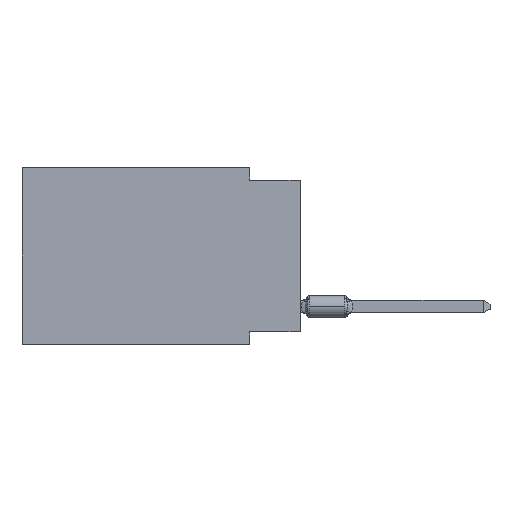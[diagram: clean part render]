
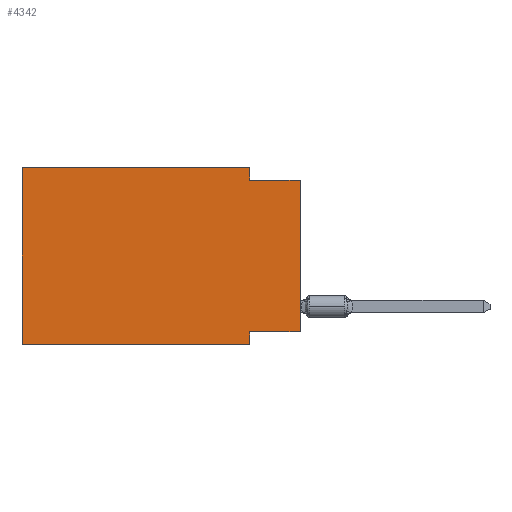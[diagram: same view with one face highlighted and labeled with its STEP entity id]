
A CAD part, left-side view. The second image highlights one B-rep face of the part: STEP entity #4342.
In plain terms, the highlighted planar face has unit normal (-1, 0, 0).
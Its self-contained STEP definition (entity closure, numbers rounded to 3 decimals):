
#394 = CARTESIAN_POINT ( 'NONE',  ( 0., 13.97, 0. ) ) ;
#446 = DIRECTION ( 'NONE',  ( 0., 1., 0. ) ) ;
#1307 = LINE ( 'NONE', #6825, #6203 ) ;
#1561 = DIRECTION ( 'NONE',  ( 0., 0., -1. ) ) ;
#2312 = CARTESIAN_POINT ( 'NONE',  ( 0., 0., -0.635 ) ) ;
#2677 = CARTESIAN_POINT ( 'NONE',  ( 0., 0., 0. ) ) ;
#3046 = EDGE_LOOP ( 'NONE', ( #17296, #5006, #12104, #15900, #17443, #9702, #17251, #3530 ) ) ;
#3286 = DIRECTION ( 'NONE',  ( 0., -1., 0. ) ) ;
#3456 = VECTOR ( 'NONE', #1561, 1000. ) ;
#3530 = ORIENTED_EDGE ( 'NONE', *, *, #16984, .F. ) ;
#3575 = CARTESIAN_POINT ( 'NONE',  ( 0., 2.54, -8.89 ) ) ;
#3631 = VERTEX_POINT ( 'NONE', #10836 ) ;
#3987 = VERTEX_POINT ( 'NONE', #11901 ) ;
#4277 = CARTESIAN_POINT ( 'NONE',  ( 0., 2.54, 0. ) ) ;
#4342 = ADVANCED_FACE ( 'NONE', ( #6666 ), #5301, .F. ) ;
#4349 = CARTESIAN_POINT ( 'NONE',  ( 0., 0., -8.255 ) ) ;
#4372 = VERTEX_POINT ( 'NONE', #14952 ) ;
#4436 = EDGE_CURVE ( 'NONE', #3631, #6353, #15126, .T. ) ;
#4737 = LINE ( 'NONE', #2312, #9221 ) ;
#4914 = VERTEX_POINT ( 'NONE', #13649 ) ;
#5006 = ORIENTED_EDGE ( 'NONE', *, *, #14986, .F. ) ;
#5114 = LINE ( 'NONE', #3575, #11708 ) ;
#5301 = PLANE ( 'NONE',  #11368 ) ;
#6203 = VECTOR ( 'NONE', #12318, 1000. ) ;
#6353 = VERTEX_POINT ( 'NONE', #12789 ) ;
#6480 = DIRECTION ( 'NONE',  ( 0., 0., -1. ) ) ;
#6558 = CARTESIAN_POINT ( 'NONE',  ( 0., 13.97, 0. ) ) ;
#6666 = FACE_OUTER_BOUND ( 'NONE', #3046, .T. ) ;
#6825 = CARTESIAN_POINT ( 'NONE',  ( 0., 13.97, -8.89 ) ) ;
#7093 = EDGE_CURVE ( 'NONE', #7919, #4914, #1307, .T. ) ;
#7183 = EDGE_CURVE ( 'NONE', #15101, #3987, #10141, .T. ) ;
#7353 = CARTESIAN_POINT ( 'NONE',  ( 0., 13.97, 0. ) ) ;
#7648 = LINE ( 'NONE', #4349, #14333 ) ;
#7919 = VERTEX_POINT ( 'NONE', #17100 ) ;
#7927 = VECTOR ( 'NONE', #8531, 1000. ) ;
#8531 = DIRECTION ( 'NONE',  ( 0., 0., 1. ) ) ;
#8983 = EDGE_CURVE ( 'NONE', #15997, #4914, #5114, .T. ) ;
#9221 = VECTOR ( 'NONE', #17374, 1000. ) ;
#9653 = CARTESIAN_POINT ( 'NONE',  ( 0., 2.54, -8.255 ) ) ;
#9702 = ORIENTED_EDGE ( 'NONE', *, *, #7093, .T. ) ;
#10141 = LINE ( 'NONE', #394, #17426 ) ;
#10621 = CARTESIAN_POINT ( 'NONE',  ( 0., 13.97, 0. ) ) ;
#10836 = CARTESIAN_POINT ( 'NONE',  ( 0., 0., -8.255 ) ) ;
#11368 = AXIS2_PLACEMENT_3D ( 'NONE', #10621, #17573, #6480 ) ;
#11708 = VECTOR ( 'NONE', #14495, 1000. ) ;
#11716 = EDGE_CURVE ( 'NONE', #7919, #15101, #17089, .T. ) ;
#11901 = CARTESIAN_POINT ( 'NONE',  ( 0., 2.54, 0. ) ) ;
#11951 = EDGE_CURVE ( 'NONE', #3987, #4372, #12483, .T. ) ;
#12104 = ORIENTED_EDGE ( 'NONE', *, *, #11951, .F. ) ;
#12318 = DIRECTION ( 'NONE',  ( 0., -1., 0. ) ) ;
#12483 = LINE ( 'NONE', #4277, #3456 ) ;
#12789 = CARTESIAN_POINT ( 'NONE',  ( 0., 0., -0.635 ) ) ;
#12850 = DIRECTION ( 'NONE',  ( 0., 0., 1. ) ) ;
#13649 = CARTESIAN_POINT ( 'NONE',  ( 0., 2.54, -8.89 ) ) ;
#14095 = VECTOR ( 'NONE', #12850, 1000. ) ;
#14333 = VECTOR ( 'NONE', #446, 1000. ) ;
#14495 = DIRECTION ( 'NONE',  ( 0., 0., -1. ) ) ;
#14952 = CARTESIAN_POINT ( 'NONE',  ( 0., 2.54, -0.635 ) ) ;
#14986 = EDGE_CURVE ( 'NONE', #4372, #6353, #4737, .T. ) ;
#15101 = VERTEX_POINT ( 'NONE', #6558 ) ;
#15126 = LINE ( 'NONE', #2677, #7927 ) ;
#15900 = ORIENTED_EDGE ( 'NONE', *, *, #7183, .F. ) ;
#15997 = VERTEX_POINT ( 'NONE', #9653 ) ;
#16984 = EDGE_CURVE ( 'NONE', #3631, #15997, #7648, .T. ) ;
#17089 = LINE ( 'NONE', #7353, #14095 ) ;
#17100 = CARTESIAN_POINT ( 'NONE',  ( 0., 13.97, -8.89 ) ) ;
#17251 = ORIENTED_EDGE ( 'NONE', *, *, #8983, .F. ) ;
#17296 = ORIENTED_EDGE ( 'NONE', *, *, #4436, .T. ) ;
#17374 = DIRECTION ( 'NONE',  ( 0., -1., 0. ) ) ;
#17426 = VECTOR ( 'NONE', #3286, 1000. ) ;
#17443 = ORIENTED_EDGE ( 'NONE', *, *, #11716, .F. ) ;
#17573 = DIRECTION ( 'NONE',  ( 1., 0., 0. ) ) ;
